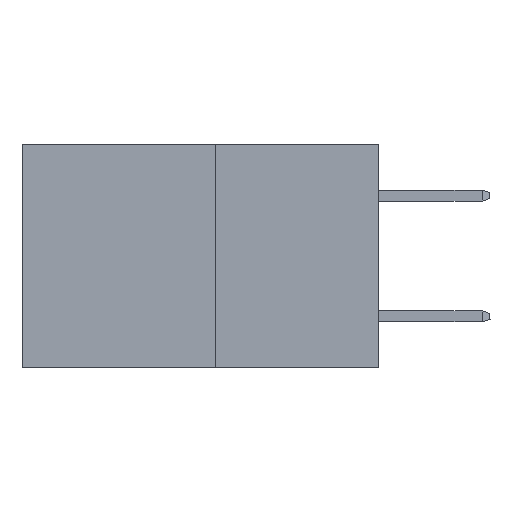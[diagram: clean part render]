
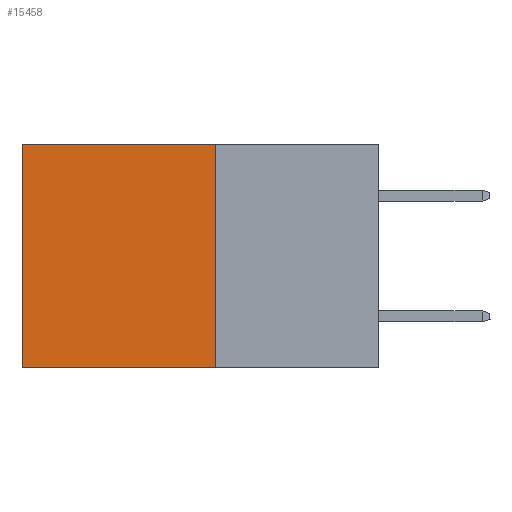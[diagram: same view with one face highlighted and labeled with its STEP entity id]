
A CAD part, left-side view. The second image highlights one B-rep face of the part: STEP entity #15458.
In plain terms, the highlighted planar face has unit normal (-1, 0, 0).
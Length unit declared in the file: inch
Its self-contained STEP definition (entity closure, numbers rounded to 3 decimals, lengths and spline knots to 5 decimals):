
#234 = CARTESIAN_POINT ( 'NONE',  ( 0.277, 0.27, 0. ) ) ;
#1330 = VERTEX_POINT ( 'NONE', #3329 ) ;
#2309 = CARTESIAN_POINT ( 'NONE',  ( 0.277, 0.27, 0. ) ) ;
#2491 = ORIENTED_EDGE ( 'NONE', *, *, #7561, .F. ) ;
#2932 = ORIENTED_EDGE ( 'NONE', *, *, #7306, .T. ) ;
#3227 = VERTEX_POINT ( 'NONE', #2309 ) ;
#3329 = CARTESIAN_POINT ( 'NONE',  ( 0.277, 0.27, -0.37 ) ) ;
#3622 = VECTOR ( 'NONE', #8462, 39.37008 ) ;
#4335 = LINE ( 'NONE', #4751, #9261 ) ;
#4751 = CARTESIAN_POINT ( 'NONE',  ( 0.277, 0.27, -0.37 ) ) ;
#4860 = FACE_OUTER_BOUND ( 'NONE', #22304, .T. ) ;
#6078 = EDGE_CURVE ( 'NONE', #9187, #10534, #8934, .T. ) ;
#7306 = EDGE_CURVE ( 'NONE', #3227, #9187, #19609, .T. ) ;
#7489 = DIRECTION ( 'NONE',  ( 0., 0., -1. ) ) ;
#7561 = EDGE_CURVE ( 'NONE', #1330, #10534, #18174, .T. ) ;
#8353 = VECTOR ( 'NONE', #20735, 39.37008 ) ;
#8462 = DIRECTION ( 'NONE',  ( 0., 1., 0. ) ) ;
#8934 = LINE ( 'NONE', #18953, #8353 ) ;
#9187 = VERTEX_POINT ( 'NONE', #23313 ) ;
#9261 = VECTOR ( 'NONE', #13904, 39.37008 ) ;
#10354 = AXIS2_PLACEMENT_3D ( 'NONE', #16559, #18358, #7489 ) ;
#10534 = VERTEX_POINT ( 'NONE', #20345 ) ;
#12649 = ORIENTED_EDGE ( 'NONE', *, *, #6078, .T. ) ;
#12971 = PLANE ( 'NONE',  #10354 ) ;
#13904 = DIRECTION ( 'NONE',  ( 0., 0., -1. ) ) ;
#15458 = ADVANCED_FACE ( 'NONE', ( #4860 ), #12971, .F. ) ;
#16559 = CARTESIAN_POINT ( 'NONE',  ( 0.277, 0.27, -0.37 ) ) ;
#17481 = CARTESIAN_POINT ( 'NONE',  ( 0.277, 0.27, -0.37 ) ) ;
#18174 = LINE ( 'NONE', #17481, #3622 ) ;
#18358 = DIRECTION ( 'NONE',  ( 1., 0., 0. ) ) ;
#18817 = EDGE_CURVE ( 'NONE', #3227, #1330, #4335, .T. ) ;
#18953 = CARTESIAN_POINT ( 'NONE',  ( 0.277, 0.59, -0.37 ) ) ;
#19609 = LINE ( 'NONE', #234, #20148 ) ;
#20148 = VECTOR ( 'NONE', #20373, 39.37008 ) ;
#20345 = CARTESIAN_POINT ( 'NONE',  ( 0.277, 0.59, -0.37 ) ) ;
#20373 = DIRECTION ( 'NONE',  ( 0., 1., 0. ) ) ;
#20735 = DIRECTION ( 'NONE',  ( 0., 0., -1. ) ) ;
#21877 = ORIENTED_EDGE ( 'NONE', *, *, #18817, .F. ) ;
#22304 = EDGE_LOOP ( 'NONE', ( #12649, #2491, #21877, #2932 ) ) ;
#23313 = CARTESIAN_POINT ( 'NONE',  ( 0.277, 0.59, 0. ) ) ;
